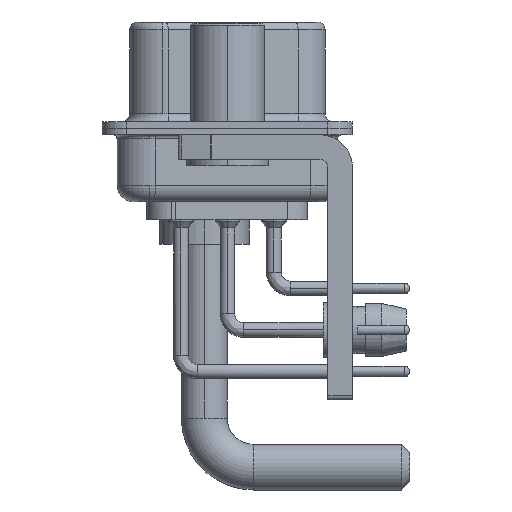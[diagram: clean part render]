
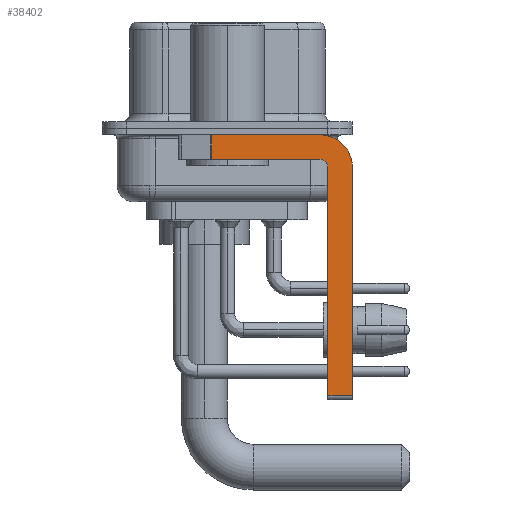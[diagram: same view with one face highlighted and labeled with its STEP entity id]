
A CAD part, left-side view. The second image highlights one B-rep face of the part: STEP entity #38402.
In plain terms, the highlighted planar face has unit normal (-1, 0, 0).
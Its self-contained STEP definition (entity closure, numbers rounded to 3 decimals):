
#268 = CARTESIAN_POINT ( 'NONE',  ( -2.9, -5.65, -2.4 ) ) ;
#924 = CARTESIAN_POINT ( 'NONE',  ( -2.9, -5.65, -1.9 ) ) ;
#1815 = CARTESIAN_POINT ( 'NONE',  ( -2.9, -6.15, -16.35 ) ) ;
#2499 = LINE ( 'NONE', #28431, #26888 ) ;
#3206 = CARTESIAN_POINT ( 'NONE',  ( -2.9, -5.65, -1.9 ) ) ;
#3469 = VECTOR ( 'NONE', #35169, 1000. ) ;
#4453 = DIRECTION ( 'NONE',  ( 0., 0., -1. ) ) ;
#5041 = DIRECTION ( 'NONE',  ( 0., 0., -1. ) ) ;
#5086 = CARTESIAN_POINT ( 'NONE',  ( -2.9, -5.65, -2.4 ) ) ;
#5398 = DIRECTION ( 'NONE',  ( 0., 0., -1. ) ) ;
#5451 = EDGE_CURVE ( 'NONE', #23181, #37185, #26508, .T. ) ;
#8099 = CIRCLE ( 'NONE', #19682, 2. ) ;
#8410 = DIRECTION ( 'NONE',  ( 1., 0., 0. ) ) ;
#8515 = EDGE_CURVE ( 'NONE', #14230, #13363, #23507, .T. ) ;
#9473 = CARTESIAN_POINT ( 'NONE',  ( -2.9, -5.65, -16.35 ) ) ;
#11413 = FACE_OUTER_BOUND ( 'NONE', #38387, .T. ) ;
#12001 = CARTESIAN_POINT ( 'NONE',  ( -2.9, -7.65, -16.35 ) ) ;
#12496 = LINE ( 'NONE', #9473, #38512 ) ;
#13178 = CARTESIAN_POINT ( 'NONE',  ( -2.9, -7.65, -2.4 ) ) ;
#13363 = VERTEX_POINT ( 'NONE', #3206 ) ;
#13528 = ORIENTED_EDGE ( 'NONE', *, *, #27383, .F. ) ;
#13701 = ORIENTED_EDGE ( 'NONE', *, *, #18086, .T. ) ;
#14230 = VERTEX_POINT ( 'NONE', #33058 ) ;
#14633 = PLANE ( 'NONE',  #17913 ) ;
#15077 = LINE ( 'NONE', #30370, #34445 ) ;
#17604 = ORIENTED_EDGE ( 'NONE', *, *, #5451, .F. ) ;
#17683 = CARTESIAN_POINT ( 'NONE',  ( -2.9, 0.978, -1.9 ) ) ;
#17913 = AXIS2_PLACEMENT_3D ( 'NONE', #32364, #8410, #5398 ) ;
#18086 = EDGE_CURVE ( 'NONE', #35258, #34887, #15077, .T. ) ;
#18518 = VECTOR ( 'NONE', #18842, 1000. ) ;
#18842 = DIRECTION ( 'NONE',  ( 0., 0., 1. ) ) ;
#19682 = AXIS2_PLACEMENT_3D ( 'NONE', #268, #22974, #4453 ) ;
#20761 = DIRECTION ( 'NONE',  ( -1., 0., 0. ) ) ;
#22618 = ORIENTED_EDGE ( 'NONE', *, *, #39197, .T. ) ;
#22713 = CARTESIAN_POINT ( 'NONE',  ( -2.9, -7.65, -2.4 ) ) ;
#22974 = DIRECTION ( 'NONE',  ( 1., 0., 0. ) ) ;
#23181 = VERTEX_POINT ( 'NONE', #13178 ) ;
#23507 = CIRCLE ( 'NONE', #35070, 0.5 ) ;
#26464 = ORIENTED_EDGE ( 'NONE', *, *, #37718, .F. ) ;
#26508 = LINE ( 'NONE', #22713, #3469 ) ;
#26748 = CARTESIAN_POINT ( 'NONE',  ( -2.9, 0.978, -0.4 ) ) ;
#26888 = VECTOR ( 'NONE', #34677, 1000. ) ;
#27383 = EDGE_CURVE ( 'NONE', #13363, #34887, #28485, .T. ) ;
#27877 = EDGE_CURVE ( 'NONE', #32213, #23181, #8099, .T. ) ;
#28277 = LINE ( 'NONE', #34723, #18518 ) ;
#28431 = CARTESIAN_POINT ( 'NONE',  ( -2.9, 3., -0.4 ) ) ;
#28485 = LINE ( 'NONE', #924, #29851 ) ;
#29851 = VECTOR ( 'NONE', #37535, 1000. ) ;
#30370 = CARTESIAN_POINT ( 'NONE',  ( -2.9, 0.978, -1.9 ) ) ;
#30410 = DIRECTION ( 'NONE',  ( 0., -1., 0. ) ) ;
#31688 = ORIENTED_EDGE ( 'NONE', *, *, #27877, .F. ) ;
#32056 = VERTEX_POINT ( 'NONE', #1815 ) ;
#32213 = VERTEX_POINT ( 'NONE', #33395 ) ;
#32364 = CARTESIAN_POINT ( 'NONE',  ( -2.9, -5.65, -2.4 ) ) ;
#32377 = ORIENTED_EDGE ( 'NONE', *, *, #37299, .F. ) ;
#33058 = CARTESIAN_POINT ( 'NONE',  ( -2.9, -6.15, -2.4 ) ) ;
#33395 = CARTESIAN_POINT ( 'NONE',  ( -2.9, -5.65, -0.4 ) ) ;
#34445 = VECTOR ( 'NONE', #5041, 1000. ) ;
#34677 = DIRECTION ( 'NONE',  ( 0., -1., 0. ) ) ;
#34723 = CARTESIAN_POINT ( 'NONE',  ( -2.9, -6.15, -16.6 ) ) ;
#34887 = VERTEX_POINT ( 'NONE', #17683 ) ;
#35070 = AXIS2_PLACEMENT_3D ( 'NONE', #5086, #20761, #35461 ) ;
#35169 = DIRECTION ( 'NONE',  ( 0., 0., -1. ) ) ;
#35258 = VERTEX_POINT ( 'NONE', #26748 ) ;
#35461 = DIRECTION ( 'NONE',  ( 0., 0., 1. ) ) ;
#37185 = VERTEX_POINT ( 'NONE', #12001 ) ;
#37299 = EDGE_CURVE ( 'NONE', #32056, #14230, #28277, .T. ) ;
#37535 = DIRECTION ( 'NONE',  ( 0., 1., 0. ) ) ;
#37718 = EDGE_CURVE ( 'NONE', #35258, #32213, #2499, .T. ) ;
#38387 = EDGE_LOOP ( 'NONE', ( #26464, #13701, #13528, #39140, #32377, #22618, #17604, #31688 ) ) ;
#38402 = ADVANCED_FACE ( 'NONE', ( #11413 ), #14633, .F. ) ;
#38512 = VECTOR ( 'NONE', #30410, 1000. ) ;
#39140 = ORIENTED_EDGE ( 'NONE', *, *, #8515, .F. ) ;
#39197 = EDGE_CURVE ( 'NONE', #32056, #37185, #12496, .T. ) ;
